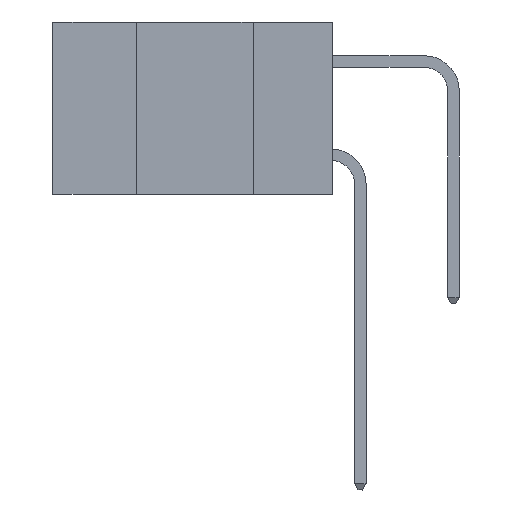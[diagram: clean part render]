
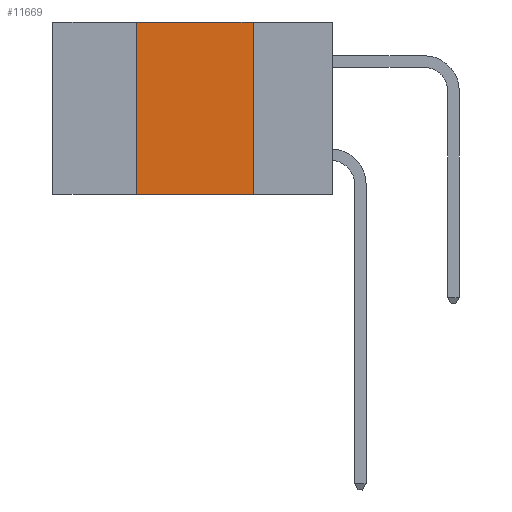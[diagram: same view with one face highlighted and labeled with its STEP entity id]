
A CAD part, left-side view. The second image highlights one B-rep face of the part: STEP entity #11669.
In plain terms, the highlighted planar face has unit normal (-1, 0, 0).
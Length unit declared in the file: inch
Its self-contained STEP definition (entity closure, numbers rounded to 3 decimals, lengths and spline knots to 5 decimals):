
#119 = EDGE_LOOP ( 'NONE', ( #10575, #13622, #5040, #11279 ) ) ;
#257 = DIRECTION ( 'NONE',  ( 0., 0., -1. ) ) ;
#282 = VERTEX_POINT ( 'NONE', #10041 ) ;
#547 = VECTOR ( 'NONE', #7885, 39.37008 ) ;
#967 = EDGE_CURVE ( 'NONE', #4757, #5633, #3575, .T. ) ;
#1768 = FACE_OUTER_BOUND ( 'NONE', #119, .T. ) ;
#2379 = EDGE_CURVE ( 'NONE', #4757, #282, #4114, .T. ) ;
#3575 = LINE ( 'NONE', #7832, #547 ) ;
#4114 = LINE ( 'NONE', #15005, #10367 ) ;
#4757 = VERTEX_POINT ( 'NONE', #12093 ) ;
#5040 = ORIENTED_EDGE ( 'NONE', *, *, #967, .F. ) ;
#5492 = VERTEX_POINT ( 'NONE', #11501 ) ;
#5633 = VERTEX_POINT ( 'NONE', #12707 ) ;
#6001 = CARTESIAN_POINT ( 'NONE',  ( 0., 0.6, 0. ) ) ;
#6621 = AXIS2_PLACEMENT_3D ( 'NONE', #13169, #14351, #7353 ) ;
#7075 = VECTOR ( 'NONE', #257, 39.37008 ) ;
#7155 = DIRECTION ( 'NONE',  ( 0., -1., 0. ) ) ;
#7353 = DIRECTION ( 'NONE',  ( 0., 0., -1. ) ) ;
#7832 = CARTESIAN_POINT ( 'NONE',  ( 0., 0.42, 0. ) ) ;
#7885 = DIRECTION ( 'NONE',  ( 0., 0., 1. ) ) ;
#8283 = EDGE_CURVE ( 'NONE', #5633, #5492, #14943, .T. ) ;
#9179 = EDGE_CURVE ( 'NONE', #5492, #282, #9895, .T. ) ;
#9602 = CARTESIAN_POINT ( 'NONE',  ( 0., 0.17, 0. ) ) ;
#9895 = LINE ( 'NONE', #9602, #7075 ) ;
#10041 = CARTESIAN_POINT ( 'NONE',  ( 0., 0.17, -0.37 ) ) ;
#10367 = VECTOR ( 'NONE', #11053, 39.37008 ) ;
#10575 = ORIENTED_EDGE ( 'NONE', *, *, #9179, .F. ) ;
#11053 = DIRECTION ( 'NONE',  ( 0., -1., 0. ) ) ;
#11279 = ORIENTED_EDGE ( 'NONE', *, *, #2379, .T. ) ;
#11501 = CARTESIAN_POINT ( 'NONE',  ( 0., 0.17, 0. ) ) ;
#11669 = ADVANCED_FACE ( 'NONE', ( #1768 ), #12021, .F. ) ;
#11848 = VECTOR ( 'NONE', #7155, 39.37008 ) ;
#12021 = PLANE ( 'NONE',  #6621 ) ;
#12093 = CARTESIAN_POINT ( 'NONE',  ( 0., 0.42, -0.37 ) ) ;
#12707 = CARTESIAN_POINT ( 'NONE',  ( 0., 0.42, 0. ) ) ;
#13169 = CARTESIAN_POINT ( 'NONE',  ( 0., 0.6, 0. ) ) ;
#13622 = ORIENTED_EDGE ( 'NONE', *, *, #8283, .F. ) ;
#14351 = DIRECTION ( 'NONE',  ( 1., 0., 0. ) ) ;
#14943 = LINE ( 'NONE', #6001, #11848 ) ;
#15005 = CARTESIAN_POINT ( 'NONE',  ( 0., 0.6, -0.37 ) ) ;
